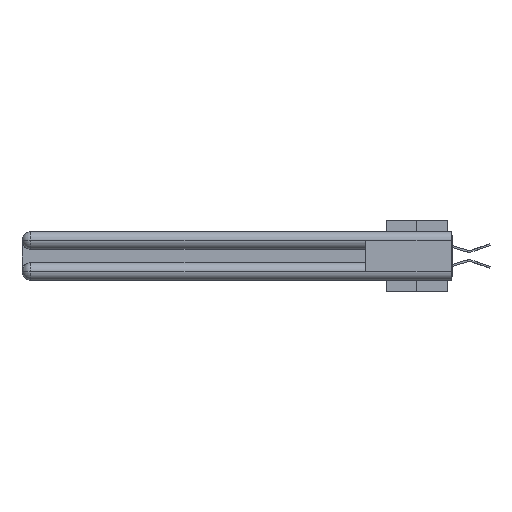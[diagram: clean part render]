
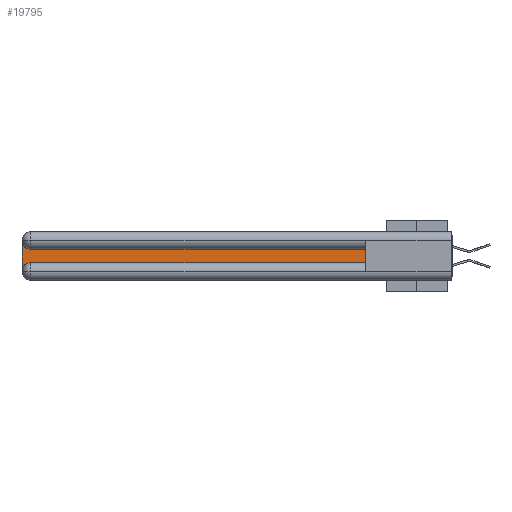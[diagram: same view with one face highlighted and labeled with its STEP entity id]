
A CAD part, left-side view. The second image highlights one B-rep face of the part: STEP entity #19795.
In plain terms, the highlighted planar face has unit normal (-1, 0, 0).
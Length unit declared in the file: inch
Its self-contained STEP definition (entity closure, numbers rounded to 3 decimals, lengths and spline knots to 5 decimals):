
#822 = CARTESIAN_POINT ( 'NONE',  ( 0.075, 0.6, -0.2175 ) ) ;
#1499 = DIRECTION ( 'NONE',  ( 1., 0., 0. ) ) ;
#1749 = VERTEX_POINT ( 'NONE', #48484 ) ;
#3278 = VECTOR ( 'NONE', #16067, 39.37008 ) ;
#3918 = CARTESIAN_POINT ( 'NONE',  ( 0.075, 0.6, -0.1225 ) ) ;
#4646 = DIRECTION ( 'NONE',  ( 0., 0., -1. ) ) ;
#5405 = VERTEX_POINT ( 'NONE', #22425 ) ;
#7181 = VERTEX_POINT ( 'NONE', #28626 ) ;
#7698 = PLANE ( 'NONE',  #36166 ) ;
#7982 = CIRCLE ( 'NONE', #22463, 0.06 ) ;
#8002 = FACE_OUTER_BOUND ( 'NONE', #43013, .T. ) ;
#9219 = CARTESIAN_POINT ( 'NONE',  ( 0.075, 2.94, -0.2775 ) ) ;
#12064 = CARTESIAN_POINT ( 'NONE',  ( 0.075, 0.6, -0.2175 ) ) ;
#12421 = AXIS2_PLACEMENT_3D ( 'NONE', #9219, #1499, #36145 ) ;
#12564 = DIRECTION ( 'NONE',  ( 1., 0., 0. ) ) ;
#12730 = ORIENTED_EDGE ( 'NONE', *, *, #31012, .T. ) ;
#12817 = DIRECTION ( 'NONE',  ( 0., 1., 0. ) ) ;
#12956 = CARTESIAN_POINT ( 'NONE',  ( 0.075, 3., -0.2775 ) ) ;
#13441 = LINE ( 'NONE', #12064, #3278 ) ;
#16067 = DIRECTION ( 'NONE',  ( 0., 0., 1. ) ) ;
#19795 = ADVANCED_FACE ( 'NONE', ( #8002 ), #7698, .F. ) ;
#20080 = DIRECTION ( 'NONE',  ( 0., 0., -1. ) ) ;
#20403 = EDGE_CURVE ( 'NONE', #21298, #1749, #34911, .T. ) ;
#20690 = EDGE_CURVE ( 'NONE', #7181, #21298, #25334, .T. ) ;
#21298 = VERTEX_POINT ( 'NONE', #12956 ) ;
#22376 = EDGE_CURVE ( 'NONE', #5405, #7181, #7982, .T. ) ;
#22425 = CARTESIAN_POINT ( 'NONE',  ( 0.075, 2.94, -0.1225 ) ) ;
#22463 = AXIS2_PLACEMENT_3D ( 'NONE', #35490, #12564, #20080 ) ;
#23406 = CARTESIAN_POINT ( 'NONE',  ( 0.075, 3., -0.2175 ) ) ;
#24483 = VECTOR ( 'NONE', #12817, 39.37008 ) ;
#25334 = LINE ( 'NONE', #23406, #44599 ) ;
#26817 = CARTESIAN_POINT ( 'NONE',  ( 0.075, 3., -0.1225 ) ) ;
#27486 = EDGE_CURVE ( 'NONE', #36614, #27903, #13441, .T. ) ;
#27903 = VERTEX_POINT ( 'NONE', #3918 ) ;
#28260 = CARTESIAN_POINT ( 'NONE',  ( 0.075, 0.6, -0.1225 ) ) ;
#28568 = DIRECTION ( 'NONE',  ( 0., -1., 0. ) ) ;
#28626 = CARTESIAN_POINT ( 'NONE',  ( 0.075, 3., -0.0625 ) ) ;
#30547 = LINE ( 'NONE', #47729, #39509 ) ;
#31012 = EDGE_CURVE ( 'NONE', #1749, #36614, #30547, .T. ) ;
#34518 = ORIENTED_EDGE ( 'NONE', *, *, #27486, .T. ) ;
#34911 = CIRCLE ( 'NONE', #12421, 0.06 ) ;
#35490 = CARTESIAN_POINT ( 'NONE',  ( 0.075, 2.94, -0.0625 ) ) ;
#36145 = DIRECTION ( 'NONE',  ( 0., 0., -1. ) ) ;
#36166 = AXIS2_PLACEMENT_3D ( 'NONE', #26817, #46146, #38011 ) ;
#36413 = ORIENTED_EDGE ( 'NONE', *, *, #36993, .T. ) ;
#36614 = VERTEX_POINT ( 'NONE', #822 ) ;
#36993 = EDGE_CURVE ( 'NONE', #27903, #5405, #46194, .T. ) ;
#38011 = DIRECTION ( 'NONE',  ( 0., 0., -1. ) ) ;
#39509 = VECTOR ( 'NONE', #28568, 39.37008 ) ;
#39744 = ORIENTED_EDGE ( 'NONE', *, *, #20403, .T. ) ;
#42973 = ORIENTED_EDGE ( 'NONE', *, *, #22376, .T. ) ;
#43013 = EDGE_LOOP ( 'NONE', ( #36413, #42973, #49425, #39744, #12730, #34518 ) ) ;
#44599 = VECTOR ( 'NONE', #4646, 39.37008 ) ;
#46146 = DIRECTION ( 'NONE',  ( 1., 0., 0. ) ) ;
#46194 = LINE ( 'NONE', #28260, #24483 ) ;
#47729 = CARTESIAN_POINT ( 'NONE',  ( 0.075, 0.6, -0.2175 ) ) ;
#48484 = CARTESIAN_POINT ( 'NONE',  ( 0.075, 2.94, -0.2175 ) ) ;
#49425 = ORIENTED_EDGE ( 'NONE', *, *, #20690, .T. ) ;
